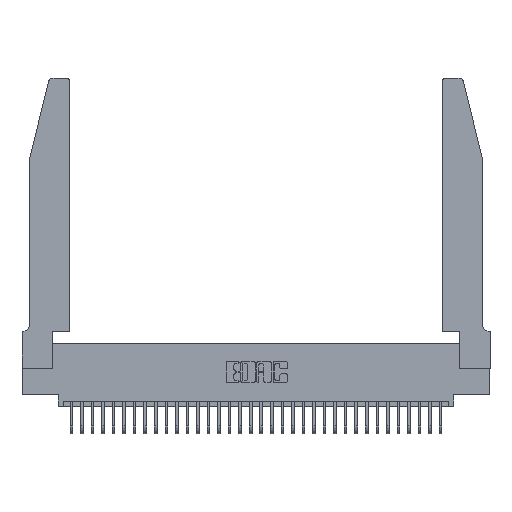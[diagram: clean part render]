
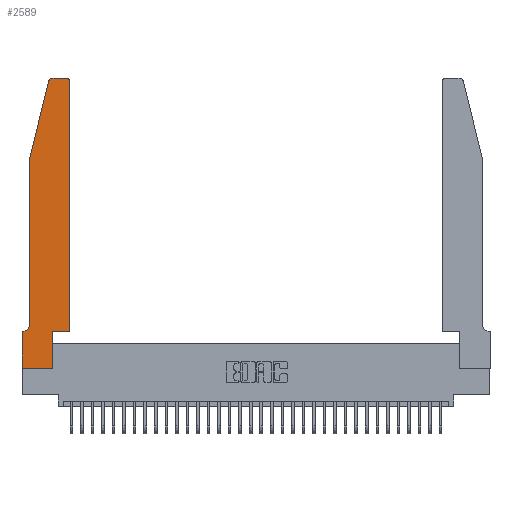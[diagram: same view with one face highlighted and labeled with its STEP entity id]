
A CAD part, top view. The second image highlights one B-rep face of the part: STEP entity #2589.
In plain terms, the highlighted planar face has unit normal (0, 0, 1).
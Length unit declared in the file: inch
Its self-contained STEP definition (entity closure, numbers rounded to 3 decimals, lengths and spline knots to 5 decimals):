
#294 = EDGE_LOOP ( 'NONE', ( #25527, #12361, #23642, #11587, #8165, #11620, #32213, #27459, #19365, #29510, #23217, #17919 ) ) ;
#568 = CARTESIAN_POINT ( 'NONE',  ( 0.4505, 0.35, 0.37 ) ) ;
#612 = EDGE_CURVE ( 'NONE', #8432, #10081, #8733, .T. ) ;
#664 = EDGE_CURVE ( 'NONE', #13795, #13043, #30210, .T. ) ;
#803 = EDGE_CURVE ( 'NONE', #13043, #13696, #18222, .T. ) ;
#1683 = PLANE ( 'NONE',  #13643 ) ;
#1706 = CARTESIAN_POINT ( 'NONE',  ( 0.2865, 0.35, 0.37 ) ) ;
#2120 = CARTESIAN_POINT ( 'NONE',  ( 0.2865, 0., 0.37 ) ) ;
#2178 = DIRECTION ( 'NONE',  ( 0., 0., 1. ) ) ;
#2288 = CARTESIAN_POINT ( 'NONE',  ( 0.0055, 0.42, 0.37 ) ) ;
#2344 = VERTEX_POINT ( 'NONE', #6144 ) ;
#2589 = ADVANCED_FACE ( 'NONE', ( #25424 ), #1683, .T. ) ;
#4725 = LINE ( 'NONE', #20254, #33070 ) ;
#4868 = VECTOR ( 'NONE', #6405, 39.37008 ) ;
#5722 = LINE ( 'NONE', #18366, #28509 ) ;
#6093 = CIRCLE ( 'NONE', #25241, 0.03 ) ;
#6144 = CARTESIAN_POINT ( 'NONE',  ( 0.25487, 2.72718, 0.37 ) ) ;
#6184 = CARTESIAN_POINT ( 'NONE',  ( 0., 0., 0.37 ) ) ;
#6265 = CARTESIAN_POINT ( 'NONE',  ( 0.284, 2.75, 0.37 ) ) ;
#6405 = DIRECTION ( 'NONE',  ( 0., -1., 0. ) ) ;
#6824 = DIRECTION ( 'NONE',  ( 1., 0., 0. ) ) ;
#6932 = DIRECTION ( 'NONE',  ( 1., 0., 0. ) ) ;
#8165 = ORIENTED_EDGE ( 'NONE', *, *, #803, .T. ) ;
#8323 = VECTOR ( 'NONE', #27272, 39.37008 ) ;
#8416 = LINE ( 'NONE', #24551, #22189 ) ;
#8432 = VERTEX_POINT ( 'NONE', #1706 ) ;
#8733 = LINE ( 'NONE', #21789, #8323 ) ;
#8842 = AXIS2_PLACEMENT_3D ( 'NONE', #23015, #12302, #17898 ) ;
#9531 = DIRECTION ( 'NONE',  ( -1., 0., 0. ) ) ;
#10081 = VERTEX_POINT ( 'NONE', #568 ) ;
#10219 = EDGE_CURVE ( 'NONE', #34296, #13617, #6093, .T. ) ;
#10897 = VERTEX_POINT ( 'NONE', #2120 ) ;
#11587 = ORIENTED_EDGE ( 'NONE', *, *, #664, .T. ) ;
#11620 = ORIENTED_EDGE ( 'NONE', *, *, #12253, .T. ) ;
#12027 = VERTEX_POINT ( 'NONE', #6265 ) ;
#12253 = EDGE_CURVE ( 'NONE', #13696, #14527, #13744, .T. ) ;
#12302 = DIRECTION ( 'NONE',  ( 0., 0., 1. ) ) ;
#12361 = ORIENTED_EDGE ( 'NONE', *, *, #22302, .T. ) ;
#12812 = CARTESIAN_POINT ( 'NONE',  ( 0., 0.35, 0.37 ) ) ;
#13043 = VERTEX_POINT ( 'NONE', #22477 ) ;
#13617 = VERTEX_POINT ( 'NONE', #20271 ) ;
#13643 = AXIS2_PLACEMENT_3D ( 'NONE', #12812, #2178, #29480 ) ;
#13646 = DIRECTION ( 'NONE',  ( 0., 1., 0. ) ) ;
#13696 = VERTEX_POINT ( 'NONE', #26069 ) ;
#13744 = LINE ( 'NONE', #17517, #14127 ) ;
#13795 = VERTEX_POINT ( 'NONE', #29169 ) ;
#14127 = VECTOR ( 'NONE', #9531, 39.37008 ) ;
#14527 = VERTEX_POINT ( 'NONE', #18226 ) ;
#14967 = LINE ( 'NONE', #17856, #21878 ) ;
#15632 = LINE ( 'NONE', #6184, #23808 ) ;
#17517 = CARTESIAN_POINT ( 'NONE',  ( 0.0755, 0.35, 0.37 ) ) ;
#17579 = EDGE_CURVE ( 'NONE', #2344, #13795, #5722, .T. ) ;
#17688 = DIRECTION ( 'NONE',  ( 0., -1., 0. ) ) ;
#17856 = CARTESIAN_POINT ( 'NONE',  ( 0.4505, 0.35, 0.37 ) ) ;
#17898 = DIRECTION ( 'NONE',  ( 1., 0., 0. ) ) ;
#17919 = ORIENTED_EDGE ( 'NONE', *, *, #10219, .T. ) ;
#18222 = CIRCLE ( 'NONE', #33419, 0.07 ) ;
#18226 = CARTESIAN_POINT ( 'NONE',  ( 0., 0.35, 0.37 ) ) ;
#18366 = CARTESIAN_POINT ( 'NONE',  ( 0.0755, 2., 0.37 ) ) ;
#19365 = ORIENTED_EDGE ( 'NONE', *, *, #30473, .T. ) ;
#20093 = EDGE_CURVE ( 'NONE', #13617, #12027, #4725, .T. ) ;
#20205 = DIRECTION ( 'NONE',  ( 0., 1., 0. ) ) ;
#20254 = CARTESIAN_POINT ( 'NONE',  ( 0.2605, 2.75, 0.37 ) ) ;
#20271 = CARTESIAN_POINT ( 'NONE',  ( 0.4205, 2.75, 0.37 ) ) ;
#20412 = DIRECTION ( 'NONE',  ( 0., 0., 1. ) ) ;
#21352 = DIRECTION ( 'NONE',  ( 0., 0., -1. ) ) ;
#21789 = CARTESIAN_POINT ( 'NONE',  ( 0.4505, 0.35, 0.37 ) ) ;
#21878 = VECTOR ( 'NONE', #20205, 39.37008 ) ;
#22189 = VECTOR ( 'NONE', #17688, 39.37008 ) ;
#22302 = EDGE_CURVE ( 'NONE', #12027, #2344, #28213, .T. ) ;
#22477 = CARTESIAN_POINT ( 'NONE',  ( 0.0755, 0.42, 0.37 ) ) ;
#22495 = CARTESIAN_POINT ( 'NONE',  ( 0., 0., 0.37 ) ) ;
#22906 = CARTESIAN_POINT ( 'NONE',  ( 0.0755, 2., 0.37 ) ) ;
#23015 = CARTESIAN_POINT ( 'NONE',  ( 0.284, 2.72, 0.37 ) ) ;
#23217 = ORIENTED_EDGE ( 'NONE', *, *, #30531, .T. ) ;
#23320 = CARTESIAN_POINT ( 'NONE',  ( 0.4205, 2.72, 0.37 ) ) ;
#23642 = ORIENTED_EDGE ( 'NONE', *, *, #17579, .T. ) ;
#23808 = VECTOR ( 'NONE', #6932, 39.37008 ) ;
#24351 = DIRECTION ( 'NONE',  ( -1., 0., 0. ) ) ;
#24551 = CARTESIAN_POINT ( 'NONE',  ( 0., 0., 0.37 ) ) ;
#24814 = CARTESIAN_POINT ( 'NONE',  ( 0.2865, 0.35, 0.37 ) ) ;
#25241 = AXIS2_PLACEMENT_3D ( 'NONE', #23320, #20412, #6824 ) ;
#25424 = FACE_OUTER_BOUND ( 'NONE', #294, .T. ) ;
#25527 = ORIENTED_EDGE ( 'NONE', *, *, #20093, .T. ) ;
#25814 = CARTESIAN_POINT ( 'NONE',  ( 0.4505, 2.72, 0.37 ) ) ;
#26069 = CARTESIAN_POINT ( 'NONE',  ( 0.0055, 0.35, 0.37 ) ) ;
#27272 = DIRECTION ( 'NONE',  ( 1., 0., 0. ) ) ;
#27459 = ORIENTED_EDGE ( 'NONE', *, *, #34404, .T. ) ;
#28213 = CIRCLE ( 'NONE', #8842, 0.03 ) ;
#28307 = VERTEX_POINT ( 'NONE', #22495 ) ;
#28509 = VECTOR ( 'NONE', #34872, 39.37008 ) ;
#28729 = VECTOR ( 'NONE', #13646, 39.37008 ) ;
#29169 = CARTESIAN_POINT ( 'NONE',  ( 0.0755, 2., 0.37 ) ) ;
#29480 = DIRECTION ( 'NONE',  ( 1., 0., 0. ) ) ;
#29510 = ORIENTED_EDGE ( 'NONE', *, *, #612, .T. ) ;
#30031 = LINE ( 'NONE', #24814, #28729 ) ;
#30210 = LINE ( 'NONE', #22906, #4868 ) ;
#30473 = EDGE_CURVE ( 'NONE', #10897, #8432, #30031, .T. ) ;
#30531 = EDGE_CURVE ( 'NONE', #10081, #34296, #14967, .T. ) ;
#32148 = EDGE_CURVE ( 'NONE', #14527, #28307, #8416, .T. ) ;
#32213 = ORIENTED_EDGE ( 'NONE', *, *, #32148, .T. ) ;
#33070 = VECTOR ( 'NONE', #34282, 39.37008 ) ;
#33419 = AXIS2_PLACEMENT_3D ( 'NONE', #2288, #21352, #24351 ) ;
#34282 = DIRECTION ( 'NONE',  ( -1., 0., 0. ) ) ;
#34296 = VERTEX_POINT ( 'NONE', #25814 ) ;
#34404 = EDGE_CURVE ( 'NONE', #28307, #10897, #15632, .T. ) ;
#34872 = DIRECTION ( 'NONE',  ( -0.239, -0.971, 0. ) ) ;
